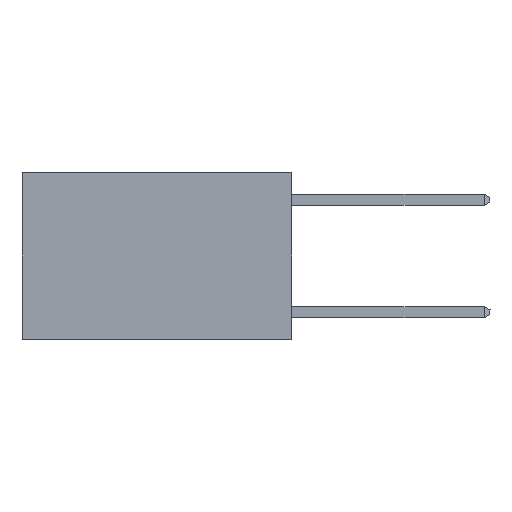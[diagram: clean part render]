
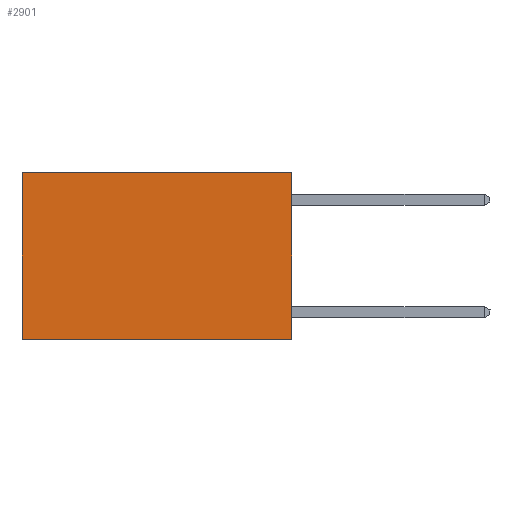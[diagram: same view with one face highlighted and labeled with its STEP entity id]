
A CAD part, left-side view. The second image highlights one B-rep face of the part: STEP entity #2901.
In plain terms, the highlighted planar face has unit normal (-1, 0, 0).
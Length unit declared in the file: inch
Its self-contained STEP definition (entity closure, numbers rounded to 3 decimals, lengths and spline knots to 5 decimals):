
#149 = VERTEX_POINT ( 'NONE', #311 ) ;
#311 = CARTESIAN_POINT ( 'NONE',  ( 0.2625, 0., 0. ) ) ;
#873 = CARTESIAN_POINT ( 'NONE',  ( 0.2625, 0., 0. ) ) ;
#967 = CARTESIAN_POINT ( 'NONE',  ( 0.2625, 0.6, -0.37 ) ) ;
#1419 = ORIENTED_EDGE ( 'NONE', *, *, #3353, .T. ) ;
#2366 = DIRECTION ( 'NONE',  ( 0., 0., -1. ) ) ;
#2521 = EDGE_CURVE ( 'NONE', #3330, #10765, #11583, .T. ) ;
#2897 = LINE ( 'NONE', #8368, #17070 ) ;
#2901 = ADVANCED_FACE ( 'NONE', ( #16447 ), #9342, .F. ) ;
#3330 = VERTEX_POINT ( 'NONE', #11456 ) ;
#3353 = EDGE_CURVE ( 'NONE', #149, #3330, #17086, .T. ) ;
#3756 = CARTESIAN_POINT ( 'NONE',  ( 0.2625, 0., -0.37 ) ) ;
#3842 = EDGE_CURVE ( 'NONE', #13302, #10765, #2897, .T. ) ;
#4216 = DIRECTION ( 'NONE',  ( 0., 1., 0. ) ) ;
#5265 = ORIENTED_EDGE ( 'NONE', *, *, #13474, .F. ) ;
#7467 = CARTESIAN_POINT ( 'NONE',  ( 0.2625, 0., 0. ) ) ;
#7964 = VECTOR ( 'NONE', #11305, 39.37008 ) ;
#8004 = VECTOR ( 'NONE', #16393, 39.37008 ) ;
#8274 = CARTESIAN_POINT ( 'NONE',  ( 0.2625, 0., 0. ) ) ;
#8368 = CARTESIAN_POINT ( 'NONE',  ( 0.2625, 0., -0.37 ) ) ;
#9342 = PLANE ( 'NONE',  #17832 ) ;
#9946 = CARTESIAN_POINT ( 'NONE',  ( 0.2625, 0.6, 0. ) ) ;
#10684 = DIRECTION ( 'NONE',  ( 1., 0., 0. ) ) ;
#10765 = VERTEX_POINT ( 'NONE', #967 ) ;
#10922 = EDGE_LOOP ( 'NONE', ( #16086, #11966, #5265, #1419 ) ) ;
#11196 = LINE ( 'NONE', #8274, #8004 ) ;
#11305 = DIRECTION ( 'NONE',  ( 0., 0., -1. ) ) ;
#11456 = CARTESIAN_POINT ( 'NONE',  ( 0.2625, 0.6, 0. ) ) ;
#11583 = LINE ( 'NONE', #9946, #7964 ) ;
#11966 = ORIENTED_EDGE ( 'NONE', *, *, #3842, .F. ) ;
#13302 = VERTEX_POINT ( 'NONE', #3756 ) ;
#13474 = EDGE_CURVE ( 'NONE', #149, #13302, #11196, .T. ) ;
#13482 = VECTOR ( 'NONE', #16966, 39.37008 ) ;
#16086 = ORIENTED_EDGE ( 'NONE', *, *, #2521, .T. ) ;
#16393 = DIRECTION ( 'NONE',  ( 0., 0., -1. ) ) ;
#16447 = FACE_OUTER_BOUND ( 'NONE', #10922, .T. ) ;
#16966 = DIRECTION ( 'NONE',  ( 0., 1., 0. ) ) ;
#17070 = VECTOR ( 'NONE', #4216, 39.37008 ) ;
#17086 = LINE ( 'NONE', #7467, #13482 ) ;
#17832 = AXIS2_PLACEMENT_3D ( 'NONE', #873, #10684, #2366 ) ;
